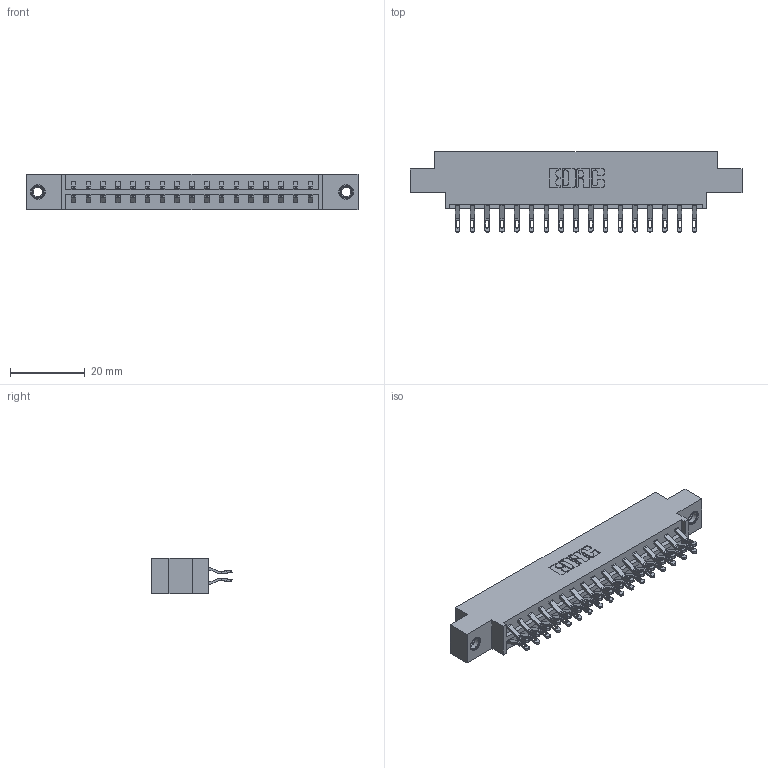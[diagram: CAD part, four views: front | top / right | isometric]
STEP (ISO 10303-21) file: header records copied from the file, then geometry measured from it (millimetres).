
FILE_DESCRIPTION (( 'STEP AP203' ), '1' );
FILE_NAME ('333-034-555-807.STEP', '2018-08-02T22:48:00', ( '' ), ( '' ), 'SwSTEP 2.0', 'SolidWorks 2016', '' );
FILE_SCHEMA (( 'CONFIG_CONTROL_DESIGN' ));
Length unit declared in the file: inch
Products named in the file (4): 345-292-001_555 Tail; 345-250-001_345-250-005-103; 333-034-555-807; 333 Part_Offset - .156 Dia - TI
Assembly tree (37 placements, depth 2):
  333-034-555-807
    333 Part_Offset - .156 Dia - TI
    345-292-001_555 Tail  x34
    345-250-001_345-250-005-103  x2
Bounding box: 88.9 x 21.47 x 9.4 mm (x, y, z)
Volume: 8699.7 mm3; surface area: 10640.3 mm2
Topology: 37 solids, 37 shells, 2150 faces, 6681 edges, 4446 vertices
Faces by surface type: plane 1262, cylinder 872, cone 12, torus 4
Entity records: 15814 total; most frequent: CARTESIAN_POINT 2671, ORIENTED_EDGE 2570, DIRECTION 2327, EDGE_CURVE 1285, LINE 1117, VECTOR 1117, VERTEX_POINT 852, AXIS2_PLACEMENT_3D 605
